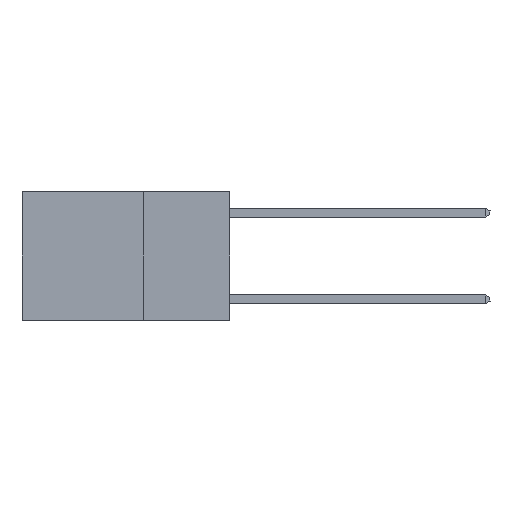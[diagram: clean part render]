
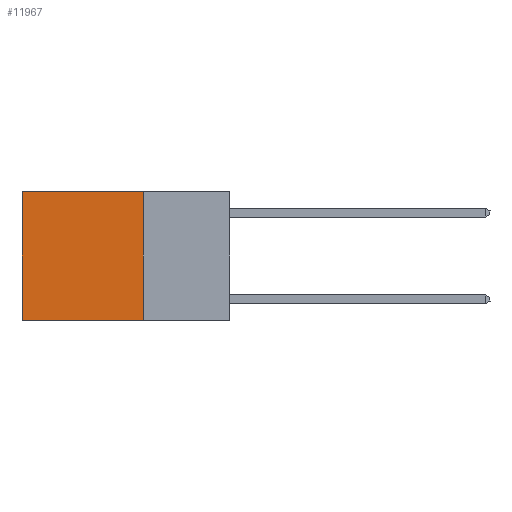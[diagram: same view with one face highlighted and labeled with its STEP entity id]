
A CAD part, left-side view. The second image highlights one B-rep face of the part: STEP entity #11967.
In plain terms, the highlighted planar face has unit normal (-1, 0, 0).
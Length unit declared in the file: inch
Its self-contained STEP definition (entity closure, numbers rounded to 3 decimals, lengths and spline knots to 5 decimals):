
#83 = ORIENTED_EDGE ( 'NONE', *, *, #694, .F. ) ;
#257 = VERTEX_POINT ( 'NONE', #15986 ) ;
#361 = DIRECTION ( 'NONE',  ( 0., 0., -1. ) ) ;
#557 = CARTESIAN_POINT ( 'NONE',  ( 0.2625, 0.25, 0. ) ) ;
#694 = EDGE_CURVE ( 'NONE', #11980, #13424, #5903, .T. ) ;
#781 = CARTESIAN_POINT ( 'NONE',  ( 0.2625, 0.25, 0. ) ) ;
#1150 = VECTOR ( 'NONE', #2152, 39.37008 ) ;
#1367 = CARTESIAN_POINT ( 'NONE',  ( 0.2625, 0.25, 0. ) ) ;
#1985 = ORIENTED_EDGE ( 'NONE', *, *, #11945, .T. ) ;
#2152 = DIRECTION ( 'NONE',  ( 0., 1., 0. ) ) ;
#2668 = ORIENTED_EDGE ( 'NONE', *, *, #2675, .T. ) ;
#2675 = EDGE_CURVE ( 'NONE', #12691, #257, #18055, .T. ) ;
#2907 = CARTESIAN_POINT ( 'NONE',  ( 0.2625, 0.6, -0.37 ) ) ;
#4280 = EDGE_LOOP ( 'NONE', ( #1985, #83, #9992, #2668 ) ) ;
#5903 = LINE ( 'NONE', #13264, #18375 ) ;
#6402 = VECTOR ( 'NONE', #17931, 39.37008 ) ;
#6925 = CARTESIAN_POINT ( 'NONE',  ( 0.2625, 0.6, 0. ) ) ;
#8440 = LINE ( 'NONE', #6925, #15870 ) ;
#8746 = CARTESIAN_POINT ( 'NONE',  ( 0.2625, 0.25, -0.37 ) ) ;
#9992 = ORIENTED_EDGE ( 'NONE', *, *, #11633, .F. ) ;
#10438 = FACE_OUTER_BOUND ( 'NONE', #4280, .T. ) ;
#11103 = CARTESIAN_POINT ( 'NONE',  ( 0.2625, 0.25, 0. ) ) ;
#11633 = EDGE_CURVE ( 'NONE', #12691, #11980, #14531, .T. ) ;
#11945 = EDGE_CURVE ( 'NONE', #257, #13424, #8440, .T. ) ;
#11967 = ADVANCED_FACE ( 'NONE', ( #10438 ), #12002, .F. ) ;
#11980 = VERTEX_POINT ( 'NONE', #8746 ) ;
#12002 = PLANE ( 'NONE',  #13621 ) ;
#12012 = DIRECTION ( 'NONE',  ( 0., 1., 0. ) ) ;
#12691 = VERTEX_POINT ( 'NONE', #11103 ) ;
#13264 = CARTESIAN_POINT ( 'NONE',  ( 0.2625, 0.25, -0.37 ) ) ;
#13424 = VERTEX_POINT ( 'NONE', #2907 ) ;
#13621 = AXIS2_PLACEMENT_3D ( 'NONE', #557, #17591, #361 ) ;
#14531 = LINE ( 'NONE', #1367, #6402 ) ;
#15339 = DIRECTION ( 'NONE',  ( 0., 0., -1. ) ) ;
#15870 = VECTOR ( 'NONE', #15339, 39.37008 ) ;
#15986 = CARTESIAN_POINT ( 'NONE',  ( 0.2625, 0.6, 0. ) ) ;
#17591 = DIRECTION ( 'NONE',  ( 1., 0., 0. ) ) ;
#17931 = DIRECTION ( 'NONE',  ( 0., 0., -1. ) ) ;
#18055 = LINE ( 'NONE', #781, #1150 ) ;
#18375 = VECTOR ( 'NONE', #12012, 39.37008 ) ;
